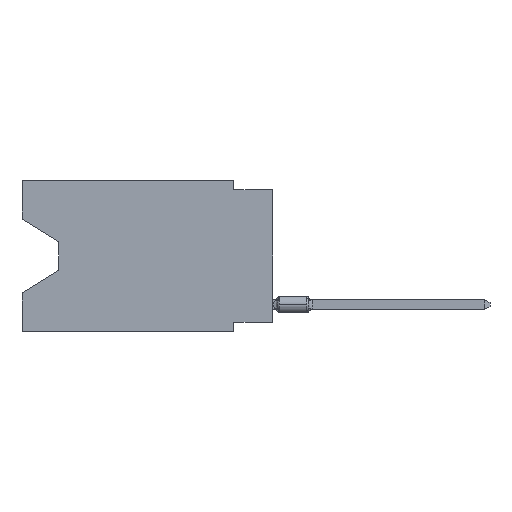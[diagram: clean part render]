
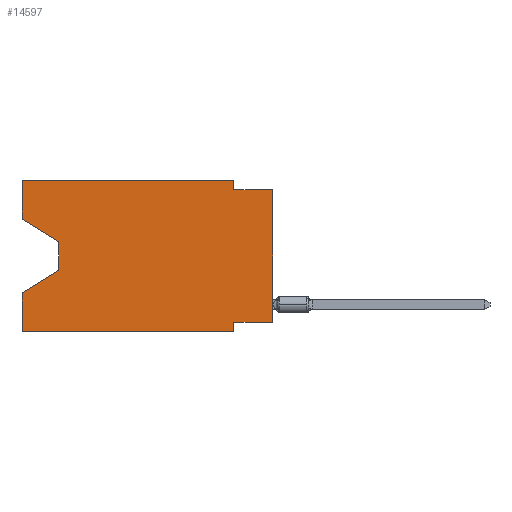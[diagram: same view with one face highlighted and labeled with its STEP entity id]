
A CAD part, left-side view. The second image highlights one B-rep face of the part: STEP entity #14597.
In plain terms, the highlighted planar face has unit normal (-1, 0, 0).
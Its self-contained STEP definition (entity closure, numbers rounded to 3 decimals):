
#243 = CARTESIAN_POINT ( 'NONE',  ( 0., 0., 0. ) ) ;
#371 = CARTESIAN_POINT ( 'NONE',  ( 0., 13.97, -4.013 ) ) ;
#773 = DIRECTION ( 'NONE',  ( 0., -0.855, -0.519 ) ) ;
#1189 = DIRECTION ( 'NONE',  ( 0., 1., 0. ) ) ;
#1372 = VERTEX_POINT ( 'NONE', #17599 ) ;
#1430 = VERTEX_POINT ( 'NONE', #20027 ) ;
#1479 = VECTOR ( 'NONE', #22949, 1000. ) ;
#1549 = VECTOR ( 'NONE', #18766, 1000. ) ;
#1765 = ORIENTED_EDGE ( 'NONE', *, *, #2584, .F. ) ;
#1792 = CARTESIAN_POINT ( 'NONE',  ( 0., 16.383, 0. ) ) ;
#2098 = ORIENTED_EDGE ( 'NONE', *, *, #8343, .T. ) ;
#2584 = EDGE_CURVE ( 'NONE', #21383, #7867, #13368, .T. ) ;
#2627 = LINE ( 'NONE', #243, #1549 ) ;
#3023 = DIRECTION ( 'NONE',  ( 0., 0.855, -0.519 ) ) ;
#3389 = CARTESIAN_POINT ( 'NONE',  ( 0., 2.54, 0. ) ) ;
#3546 = EDGE_CURVE ( 'NONE', #22687, #10842, #12585, .T. ) ;
#3675 = LINE ( 'NONE', #17626, #12742 ) ;
#3753 = EDGE_CURVE ( 'NONE', #10842, #20202, #13120, .T. ) ;
#3777 = CARTESIAN_POINT ( 'NONE',  ( 0., 16.383, -7.36 ) ) ;
#4130 = VECTOR ( 'NONE', #9947, 1000. ) ;
#4207 = ORIENTED_EDGE ( 'NONE', *, *, #16078, .T. ) ;
#4674 = LINE ( 'NONE', #21155, #6287 ) ;
#5294 = VECTOR ( 'NONE', #1189, 1000. ) ;
#5453 = DIRECTION ( 'NONE',  ( 1., 0., 0. ) ) ;
#5696 = FACE_OUTER_BOUND ( 'NONE', #6396, .T. ) ;
#5868 = VECTOR ( 'NONE', #21830, 1000. ) ;
#6204 = VERTEX_POINT ( 'NONE', #12813 ) ;
#6287 = VECTOR ( 'NONE', #773, 1000. ) ;
#6396 = EDGE_LOOP ( 'NONE', ( #6891, #11168, #13260, #11433, #2098, #8402, #8815, #4207, #24094, #25269, #1765, #20197 ) ) ;
#6578 = AXIS2_PLACEMENT_3D ( 'NONE', #1792, #5453, #16023 ) ;
#6891 = ORIENTED_EDGE ( 'NONE', *, *, #20223, .T. ) ;
#7627 = LINE ( 'NONE', #13926, #11774 ) ;
#7867 = VERTEX_POINT ( 'NONE', #3389 ) ;
#8069 = LINE ( 'NONE', #20540, #9559 ) ;
#8343 = EDGE_CURVE ( 'NONE', #1430, #20246, #15320, .T. ) ;
#8402 = ORIENTED_EDGE ( 'NONE', *, *, #18973, .F. ) ;
#8508 = VERTEX_POINT ( 'NONE', #17705 ) ;
#8815 = ORIENTED_EDGE ( 'NONE', *, *, #22928, .F. ) ;
#9559 = VECTOR ( 'NONE', #14514, 1000. ) ;
#9947 = DIRECTION ( 'NONE',  ( 0., -1., 0. ) ) ;
#10842 = VERTEX_POINT ( 'NONE', #15008 ) ;
#11168 = ORIENTED_EDGE ( 'NONE', *, *, #3546, .T. ) ;
#11400 = CARTESIAN_POINT ( 'NONE',  ( 0., 16.383, 0. ) ) ;
#11433 = ORIENTED_EDGE ( 'NONE', *, *, #16316, .F. ) ;
#11512 = LINE ( 'NONE', #23560, #5294 ) ;
#11591 = PLANE ( 'NONE',  #6578 ) ;
#11774 = VECTOR ( 'NONE', #23565, 1000. ) ;
#11866 = DIRECTION ( 'NONE',  ( 0., 0., -1. ) ) ;
#12015 = DIRECTION ( 'NONE',  ( 0., 0., 1. ) ) ;
#12351 = CARTESIAN_POINT ( 'NONE',  ( 0., 13.97, -4.013 ) ) ;
#12585 = LINE ( 'NONE', #371, #13998 ) ;
#12742 = VECTOR ( 'NONE', #11866, 1000. ) ;
#12813 = CARTESIAN_POINT ( 'NONE',  ( 0., 2.54, -0.635 ) ) ;
#13100 = EDGE_CURVE ( 'NONE', #8508, #21383, #26507, .T. ) ;
#13120 = LINE ( 'NONE', #21293, #25978 ) ;
#13260 = ORIENTED_EDGE ( 'NONE', *, *, #3753, .T. ) ;
#13368 = LINE ( 'NONE', #14132, #4130 ) ;
#13926 = CARTESIAN_POINT ( 'NONE',  ( 0., 0., -0.635 ) ) ;
#13998 = VECTOR ( 'NONE', #20627, 1000. ) ;
#14132 = CARTESIAN_POINT ( 'NONE',  ( 0., 16.383, 0. ) ) ;
#14514 = DIRECTION ( 'NONE',  ( 0., 0., -1. ) ) ;
#14597 = ADVANCED_FACE ( 'NONE', ( #5696 ), #11591, .F. ) ;
#14706 = CARTESIAN_POINT ( 'NONE',  ( 0., 2.54, -9.271 ) ) ;
#14867 = VERTEX_POINT ( 'NONE', #17486 ) ;
#15008 = CARTESIAN_POINT ( 'NONE',  ( 0., 13.97, -5.893 ) ) ;
#15320 = LINE ( 'NONE', #17307, #1479 ) ;
#15674 = CARTESIAN_POINT ( 'NONE',  ( 0., 16.383, 0. ) ) ;
#16023 = DIRECTION ( 'NONE',  ( 0., 0., -1. ) ) ;
#16078 = EDGE_CURVE ( 'NONE', #1372, #14867, #2627, .T. ) ;
#16316 = EDGE_CURVE ( 'NONE', #1430, #20202, #21819, .T. ) ;
#16811 = EDGE_CURVE ( 'NONE', #7867, #6204, #3675, .T. ) ;
#17307 = CARTESIAN_POINT ( 'NONE',  ( 0., 16.383, -9.906 ) ) ;
#17486 = CARTESIAN_POINT ( 'NONE',  ( 0., 0., -0.635 ) ) ;
#17599 = CARTESIAN_POINT ( 'NONE',  ( 0., 0., -9.271 ) ) ;
#17626 = CARTESIAN_POINT ( 'NONE',  ( 0., 2.54, 0. ) ) ;
#17705 = CARTESIAN_POINT ( 'NONE',  ( 0., 16.383, -2.546 ) ) ;
#18200 = CARTESIAN_POINT ( 'NONE',  ( 0., 16.383, 0. ) ) ;
#18766 = DIRECTION ( 'NONE',  ( 0., 0., 1. ) ) ;
#18973 = EDGE_CURVE ( 'NONE', #23199, #20246, #8069, .T. ) ;
#20027 = CARTESIAN_POINT ( 'NONE',  ( 0., 16.383, -9.906 ) ) ;
#20197 = ORIENTED_EDGE ( 'NONE', *, *, #13100, .F. ) ;
#20202 = VERTEX_POINT ( 'NONE', #3777 ) ;
#20223 = EDGE_CURVE ( 'NONE', #8508, #22687, #4674, .T. ) ;
#20246 = VERTEX_POINT ( 'NONE', #23039 ) ;
#20540 = CARTESIAN_POINT ( 'NONE',  ( 0., 2.54, -9.906 ) ) ;
#20627 = DIRECTION ( 'NONE',  ( 0., 0., -1. ) ) ;
#21155 = CARTESIAN_POINT ( 'NONE',  ( 0., 16.383, -2.546 ) ) ;
#21293 = CARTESIAN_POINT ( 'NONE',  ( 0., 13.97, -5.893 ) ) ;
#21383 = VERTEX_POINT ( 'NONE', #11400 ) ;
#21819 = LINE ( 'NONE', #18200, #24238 ) ;
#21830 = DIRECTION ( 'NONE',  ( 0., 0., 1. ) ) ;
#22687 = VERTEX_POINT ( 'NONE', #12351 ) ;
#22928 = EDGE_CURVE ( 'NONE', #1372, #23199, #11512, .T. ) ;
#22949 = DIRECTION ( 'NONE',  ( 0., -1., 0. ) ) ;
#23039 = CARTESIAN_POINT ( 'NONE',  ( 0., 2.54, -9.906 ) ) ;
#23199 = VERTEX_POINT ( 'NONE', #14706 ) ;
#23560 = CARTESIAN_POINT ( 'NONE',  ( 0., 0., -9.271 ) ) ;
#23565 = DIRECTION ( 'NONE',  ( 0., -1., 0. ) ) ;
#24094 = ORIENTED_EDGE ( 'NONE', *, *, #24170, .F. ) ;
#24170 = EDGE_CURVE ( 'NONE', #6204, #14867, #7627, .T. ) ;
#24238 = VECTOR ( 'NONE', #12015, 1000. ) ;
#25269 = ORIENTED_EDGE ( 'NONE', *, *, #16811, .F. ) ;
#25978 = VECTOR ( 'NONE', #3023, 1000. ) ;
#26507 = LINE ( 'NONE', #15674, #5868 ) ;
